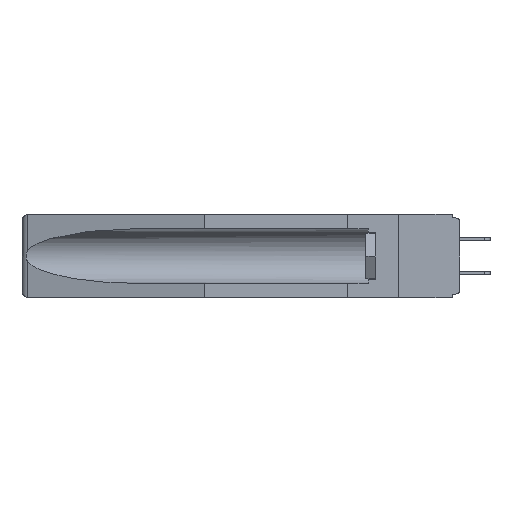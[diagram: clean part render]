
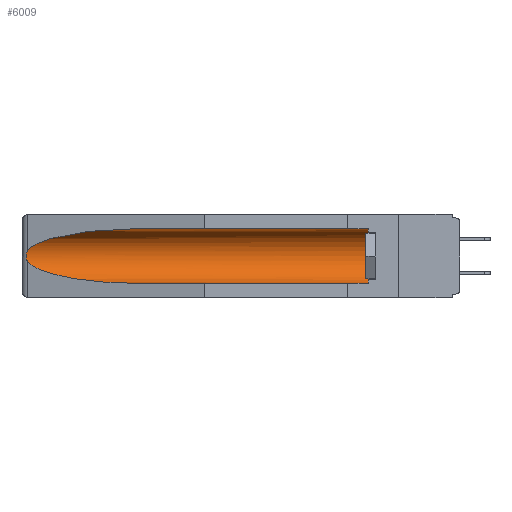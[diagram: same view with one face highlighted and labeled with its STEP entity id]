
A CAD part, left-side view. The second image highlights one B-rep face of the part: STEP entity #6009.
In plain terms, the highlighted cylindrical face has radius 2.857 mm (diameter 5.715 mm), a partial arc.
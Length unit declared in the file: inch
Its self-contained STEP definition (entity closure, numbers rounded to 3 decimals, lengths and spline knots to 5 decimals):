
#316 = CARTESIAN_POINT ( 'NONE',  ( 0.26597, 1.52961, -0.15275 ) ) ;
#558 = ORIENTED_EDGE ( 'NONE', *, *, #23492, .T. ) ;
#575 = LINE ( 'NONE', #9692, #9561 ) ;
#1293 = CARTESIAN_POINT ( 'NONE',  ( 0.155, 0.126, -0.284 ) ) ;
#1502 = ORIENTED_EDGE ( 'NONE', *, *, #21943, .T. ) ;
#2065 = B_SPLINE_CURVE_WITH_KNOTS ( 'NONE', 3,
 ( #4229, #316, #2482, #21499, #17800, #8241, #23508, #12109, #5057, #22338 ),
 .UNSPECIFIED., .F., .F.,
 ( 4, 2, 2, 2, 4 ),
 ( 0., 0.00029, 0.00058, 0.00087, 0.00117 ),
 .UNSPECIFIED. ) ;
#2482 = CARTESIAN_POINT ( 'NONE',  ( 0.26654, 1.53092, -0.15636 ) ) ;
#2622 = LINE ( 'NONE', #3209, #10712 ) ;
#2809 = CARTESIAN_POINT ( 'NONE',  ( 0.25451, 1.48313, -0.24835 ) ) ;
#3209 = CARTESIAN_POINT ( 'NONE',  ( 0.155, -0.30754, -0.059 ) ) ;
#4118 = VERTEX_POINT ( 'NONE', #9115 ) ;
#4229 = CARTESIAN_POINT ( 'NONE',  ( 0.26537, 1.52718, -0.14972 ) ) ;
#4613 = CARTESIAN_POINT ( 'NONE',  ( 0.155, 1.07973, -0.284 ) ) ;
#4817 = CARTESIAN_POINT ( 'NONE',  ( 0.21114, 1.30732, -0.284 ) ) ;
#5056 = CYLINDRICAL_SURFACE ( 'NONE', #13529, 0.1125 ) ;
#5057 = CARTESIAN_POINT ( 'NONE',  ( 0.26597, 1.5296, -0.19026 ) ) ;
#5248 = EDGE_CURVE ( 'NONE', #4118, #13056, #10923, .T. ) ;
#5419 = CIRCLE ( 'NONE', #15579, 0.1125 ) ;
#5798 = CARTESIAN_POINT ( 'NONE',  ( 0.155, 0.126, -0.059 ) ) ;
#5958 = EDGE_CURVE ( 'NONE', #9176, #13056, #575, .T. ) ;
#5976 = EDGE_CURVE ( 'NONE', #11141, #20697, #14063, .T. ) ;
#6009 = ADVANCED_FACE ( 'NONE', ( #20309 ), #5056, .F. ) ;
#8086 = CARTESIAN_POINT ( 'NONE',  ( 0.21114, 1.30732, -0.059 ) ) ;
#8166 = CARTESIAN_POINT ( 'NONE',  ( 0.155, -0.30754, -0.1715 ) ) ;
#8241 = CARTESIAN_POINT ( 'NONE',  ( 0.2675, 1.53308, -0.17534 ) ) ;
#9115 = CARTESIAN_POINT ( 'NONE',  ( 0.26537, 1.52718, -0.19328 ) ) ;
#9176 = VERTEX_POINT ( 'NONE', #1293 ) ;
#9561 = VECTOR ( 'NONE', #21262, 39.37008 ) ;
#9603 = CARTESIAN_POINT ( 'NONE',  ( 0.155, 0.126, -0.1715 ) ) ;
#9692 = CARTESIAN_POINT ( 'NONE',  ( 0.155, -0.30754, -0.284 ) ) ;
#10712 = VECTOR ( 'NONE', #22304, 39.37008 ) ;
#10923 =( BOUNDED_CURVE ( )  B_SPLINE_CURVE ( 3, ( #18044, #2809, #4817, #12690 ),
 .UNSPECIFIED., .F., .F. ) 
 B_SPLINE_CURVE_WITH_KNOTS ( ( 4, 4 ),
 ( 0.1948, 1.5708 ),
 .UNSPECIFIED. ) 
 CURVE ( )  GEOMETRIC_REPRESENTATION_ITEM ( )  RATIONAL_B_SPLINE_CURVE ( ( 1., 0.848, 0.848, 1. ) ) 
 REPRESENTATION_ITEM ( '' )  );
#11141 = VERTEX_POINT ( 'NONE', #19721 ) ;
#11509 = EDGE_CURVE ( 'NONE', #9176, #18392, #5419, .T. ) ;
#11879 = ORIENTED_EDGE ( 'NONE', *, *, #5976, .T. ) ;
#12044 = DIRECTION ( 'NONE',  ( 0., 0., 1. ) ) ;
#12109 = CARTESIAN_POINT ( 'NONE',  ( 0.26655, 1.53094, -0.18657 ) ) ;
#12690 = CARTESIAN_POINT ( 'NONE',  ( 0.155, 1.07973, -0.284 ) ) ;
#13056 = VERTEX_POINT ( 'NONE', #4613 ) ;
#13226 = DIRECTION ( 'NONE',  ( 0., 0., 1. ) ) ;
#13529 = AXIS2_PLACEMENT_3D ( 'NONE', #8166, #21520, #12044 ) ;
#13812 = CARTESIAN_POINT ( 'NONE',  ( 0.155, 1.07973, -0.059 ) ) ;
#14063 =( BOUNDED_CURVE ( )  B_SPLINE_CURVE ( 3, ( #13812, #8086, #23198, #17330 ),
 .UNSPECIFIED., .F., .T. ) 
 B_SPLINE_CURVE_WITH_KNOTS ( ( 4, 4 ),
 ( 4.71239, 6.08839 ),
 .UNSPECIFIED. ) 
 CURVE ( )  GEOMETRIC_REPRESENTATION_ITEM ( )  RATIONAL_B_SPLINE_CURVE ( ( 1., 0.848, 0.848, 1. ) ) 
 REPRESENTATION_ITEM ( '' )  );
#14136 = ORIENTED_EDGE ( 'NONE', *, *, #11509, .T. ) ;
#14962 = CARTESIAN_POINT ( 'NONE',  ( 0.26537, 1.52718, -0.14972 ) ) ;
#15579 = AXIS2_PLACEMENT_3D ( 'NONE', #9603, #22772, #13226 ) ;
#17330 = CARTESIAN_POINT ( 'NONE',  ( 0.26537, 1.52718, -0.14972 ) ) ;
#17447 = ORIENTED_EDGE ( 'NONE', *, *, #5958, .F. ) ;
#17800 = CARTESIAN_POINT ( 'NONE',  ( 0.2675, 1.53308, -0.16763 ) ) ;
#17913 = EDGE_LOOP ( 'NONE', ( #11879, #558, #22187, #17447, #14136, #1502 ) ) ;
#18044 = CARTESIAN_POINT ( 'NONE',  ( 0.26537, 1.52718, -0.19328 ) ) ;
#18392 = VERTEX_POINT ( 'NONE', #5798 ) ;
#19721 = CARTESIAN_POINT ( 'NONE',  ( 0.155, 1.07973, -0.059 ) ) ;
#20309 = FACE_OUTER_BOUND ( 'NONE', #17913, .T. ) ;
#20697 = VERTEX_POINT ( 'NONE', #14962 ) ;
#21262 = DIRECTION ( 'NONE',  ( 0., 1., 0. ) ) ;
#21499 = CARTESIAN_POINT ( 'NONE',  ( 0.2673, 1.5327, -0.16383 ) ) ;
#21520 = DIRECTION ( 'NONE',  ( 0., 1., 0. ) ) ;
#21943 = EDGE_CURVE ( 'NONE', #18392, #11141, #2622, .T. ) ;
#22187 = ORIENTED_EDGE ( 'NONE', *, *, #5248, .T. ) ;
#22304 = DIRECTION ( 'NONE',  ( 0., 1., 0. ) ) ;
#22338 = CARTESIAN_POINT ( 'NONE',  ( 0.26537, 1.52718, -0.19328 ) ) ;
#22772 = DIRECTION ( 'NONE',  ( 0., -1., 0. ) ) ;
#23198 = CARTESIAN_POINT ( 'NONE',  ( 0.25451, 1.48313, -0.09465 ) ) ;
#23492 = EDGE_CURVE ( 'NONE', #20697, #4118, #2065, .T. ) ;
#23508 = CARTESIAN_POINT ( 'NONE',  ( 0.2673, 1.53269, -0.17917 ) ) ;
